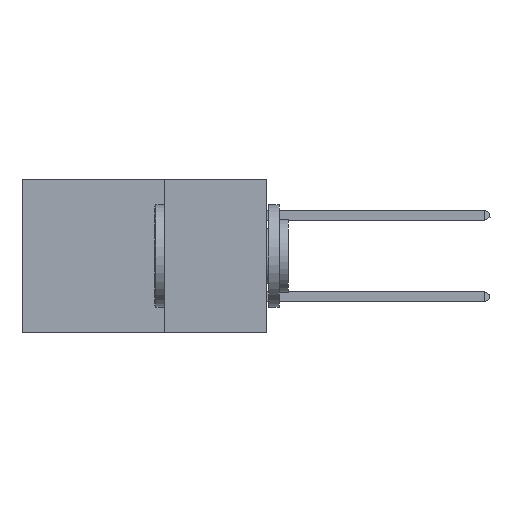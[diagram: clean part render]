
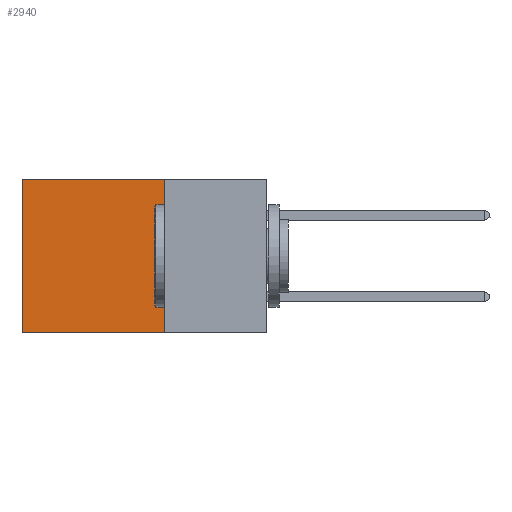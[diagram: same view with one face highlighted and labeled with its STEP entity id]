
A CAD part, left-side view. The second image highlights one B-rep face of the part: STEP entity #2940.
In plain terms, the highlighted planar face has unit normal (-1, 0, 0).
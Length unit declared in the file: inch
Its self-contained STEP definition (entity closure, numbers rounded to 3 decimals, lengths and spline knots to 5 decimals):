
#189 = CARTESIAN_POINT ( 'NONE',  ( 0.2875, 0.25, -0.375 ) ) ;
#425 = LINE ( 'NONE', #1921, #5286 ) ;
#609 = CARTESIAN_POINT ( 'NONE',  ( 0.2875, 0.25, 0. ) ) ;
#657 = CARTESIAN_POINT ( 'NONE',  ( 0.2875, 0.25, -0.375 ) ) ;
#727 = CARTESIAN_POINT ( 'NONE',  ( 0.2875, 0.6, 0. ) ) ;
#766 = EDGE_CURVE ( 'NONE', #8330, #4747, #8552, .T. ) ;
#996 = EDGE_CURVE ( 'NONE', #1119, #5463, #8093, .T. ) ;
#1119 = VERTEX_POINT ( 'NONE', #189 ) ;
#1160 = FACE_OUTER_BOUND ( 'NONE', #3878, .T. ) ;
#1685 = CARTESIAN_POINT ( 'NONE',  ( 0.2875, 0.25, 0. ) ) ;
#1921 = CARTESIAN_POINT ( 'NONE',  ( 0.2875, 0.6, -0.375 ) ) ;
#2504 = ORIENTED_EDGE ( 'NONE', *, *, #6925, .T. ) ;
#2596 = CARTESIAN_POINT ( 'NONE',  ( 0.2875, 0.6, -0.375 ) ) ;
#2846 = VECTOR ( 'NONE', #3470, 39.37008 ) ;
#2940 = ADVANCED_FACE ( 'NONE', ( #1160 ), #5455, .F. ) ;
#3470 = DIRECTION ( 'NONE',  ( 0., 1., 0. ) ) ;
#3694 = CARTESIAN_POINT ( 'NONE',  ( 0.2875, 0.25, -0.375 ) ) ;
#3878 = EDGE_LOOP ( 'NONE', ( #2504, #8005, #6873, #7543 ) ) ;
#4091 = DIRECTION ( 'NONE',  ( 0., 0., -1. ) ) ;
#4189 = VECTOR ( 'NONE', #5043, 39.37008 ) ;
#4678 = CARTESIAN_POINT ( 'NONE',  ( 0.2875, 0.25, -0.375 ) ) ;
#4747 = VERTEX_POINT ( 'NONE', #727 ) ;
#5043 = DIRECTION ( 'NONE',  ( 0., 0., -1. ) ) ;
#5120 = AXIS2_PLACEMENT_3D ( 'NONE', #4678, #5356, #4091 ) ;
#5286 = VECTOR ( 'NONE', #5534, 39.37008 ) ;
#5356 = DIRECTION ( 'NONE',  ( 1., 0., 0. ) ) ;
#5455 = PLANE ( 'NONE',  #5120 ) ;
#5463 = VERTEX_POINT ( 'NONE', #2596 ) ;
#5534 = DIRECTION ( 'NONE',  ( 0., 0., -1. ) ) ;
#6064 = LINE ( 'NONE', #3694, #4189 ) ;
#6609 = EDGE_CURVE ( 'NONE', #8330, #1119, #6064, .T. ) ;
#6873 = ORIENTED_EDGE ( 'NONE', *, *, #6609, .F. ) ;
#6925 = EDGE_CURVE ( 'NONE', #4747, #5463, #425, .T. ) ;
#7543 = ORIENTED_EDGE ( 'NONE', *, *, #766, .T. ) ;
#7990 = VECTOR ( 'NONE', #8546, 39.37008 ) ;
#8005 = ORIENTED_EDGE ( 'NONE', *, *, #996, .F. ) ;
#8093 = LINE ( 'NONE', #657, #7990 ) ;
#8330 = VERTEX_POINT ( 'NONE', #1685 ) ;
#8546 = DIRECTION ( 'NONE',  ( 0., 1., 0. ) ) ;
#8552 = LINE ( 'NONE', #609, #2846 ) ;
